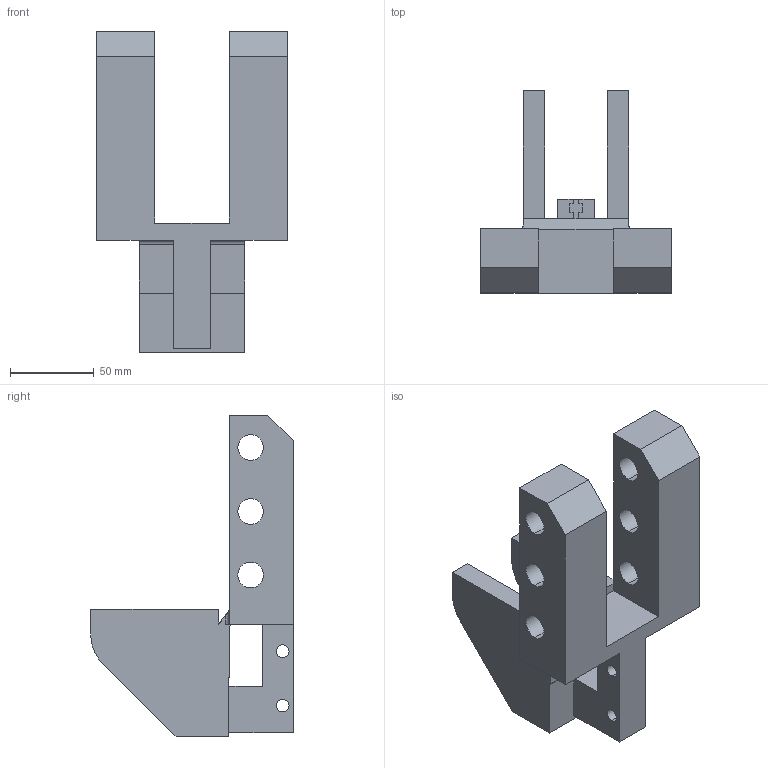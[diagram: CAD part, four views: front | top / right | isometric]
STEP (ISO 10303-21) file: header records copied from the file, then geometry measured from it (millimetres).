
FILE_DESCRIPTION (( 'STEP AP214' ), '1' );
FILE_NAME ('receiver_frame.STEP', '2013-09-07T19:04:17', ( '' ), ( '' ), 'SwSTEP 2.0', 'SolidWorks 2013', '' );
FILE_SCHEMA (( 'AUTOMOTIVE_DESIGN' ));
Length unit declared in the file: inch
Products named in the file (1): receiver_frame
Bounding box: 113.54 x 120.65 x 191.67 mm (x, y, z)
Volume: 478594.5 mm3; surface area: 90985.2 mm2
Topology: 1 solids, 1 shells, 80 faces, 241 edges, 160 vertices
Faces by surface type: plane 59, cylinder 21
Entity records: 2769 total; most frequent: CARTESIAN_POINT 488, ORIENTED_EDGE 482, DIRECTION 441, EDGE_CURVE 241, VECTOR 199, LINE 199, VERTEX_POINT 160, AXIS2_PLACEMENT_3D 121
